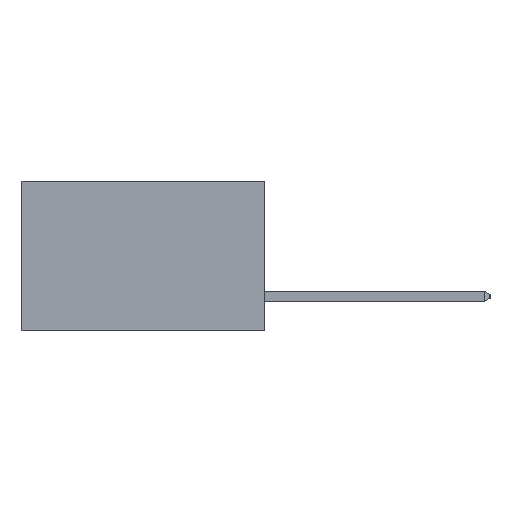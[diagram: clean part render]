
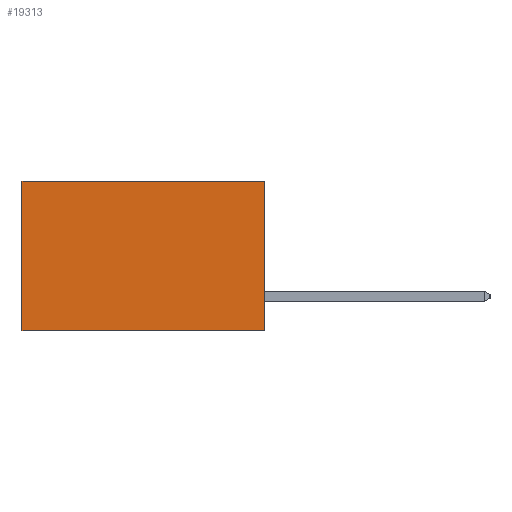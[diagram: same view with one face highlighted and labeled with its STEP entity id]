
A CAD part, left-side view. The second image highlights one B-rep face of the part: STEP entity #19313.
In plain terms, the highlighted planar face has unit normal (-1, 0, 0).
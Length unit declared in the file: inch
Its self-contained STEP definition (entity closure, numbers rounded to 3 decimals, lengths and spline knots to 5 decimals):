
#347 = ORIENTED_EDGE ( 'NONE', *, *, #15034, .F. ) ;
#660 = CARTESIAN_POINT ( 'NONE',  ( 0.2615, 0., -0.37 ) ) ;
#1065 = CARTESIAN_POINT ( 'NONE',  ( 0.2615, 0., -0.37 ) ) ;
#1078 = LINE ( 'NONE', #9106, #4583 ) ;
#1661 = EDGE_LOOP ( 'NONE', ( #18837, #2017, #347, #2575 ) ) ;
#2017 = ORIENTED_EDGE ( 'NONE', *, *, #21626, .F. ) ;
#2575 = ORIENTED_EDGE ( 'NONE', *, *, #17788, .T. ) ;
#3589 = VERTEX_POINT ( 'NONE', #18928 ) ;
#3694 = CARTESIAN_POINT ( 'NONE',  ( 0.2615, 0., 0. ) ) ;
#4120 = PLANE ( 'NONE',  #16615 ) ;
#4200 = DIRECTION ( 'NONE',  ( 1., 0., 0. ) ) ;
#4490 = CARTESIAN_POINT ( 'NONE',  ( 0.2615, 0., -0.37 ) ) ;
#4583 = VECTOR ( 'NONE', #10877, 39.37008 ) ;
#5473 = CARTESIAN_POINT ( 'NONE',  ( 0.2615, 0., 0. ) ) ;
#8933 = VECTOR ( 'NONE', #14797, 39.37008 ) ;
#9106 = CARTESIAN_POINT ( 'NONE',  ( 0.2615, 0., -0.37 ) ) ;
#9468 = LINE ( 'NONE', #4490, #8933 ) ;
#9940 = CARTESIAN_POINT ( 'NONE',  ( 0.2615, 0.6, 0. ) ) ;
#10675 = VECTOR ( 'NONE', #12567, 39.37008 ) ;
#10877 = DIRECTION ( 'NONE',  ( 0., 0., -1. ) ) ;
#12567 = DIRECTION ( 'NONE',  ( 0., 0., -1. ) ) ;
#13395 = VERTEX_POINT ( 'NONE', #3694 ) ;
#13861 = VERTEX_POINT ( 'NONE', #1065 ) ;
#14797 = DIRECTION ( 'NONE',  ( 0., 1., 0. ) ) ;
#15034 = EDGE_CURVE ( 'NONE', #13395, #13861, #1078, .T. ) ;
#15559 = LINE ( 'NONE', #5473, #19456 ) ;
#15735 = LINE ( 'NONE', #20854, #10675 ) ;
#16218 = DIRECTION ( 'NONE',  ( 0., 0., -1. ) ) ;
#16615 = AXIS2_PLACEMENT_3D ( 'NONE', #660, #4200, #16218 ) ;
#17788 = EDGE_CURVE ( 'NONE', #13395, #18881, #15559, .T. ) ;
#18837 = ORIENTED_EDGE ( 'NONE', *, *, #19802, .T. ) ;
#18881 = VERTEX_POINT ( 'NONE', #9940 ) ;
#18928 = CARTESIAN_POINT ( 'NONE',  ( 0.2615, 0.6, -0.37 ) ) ;
#19113 = DIRECTION ( 'NONE',  ( 0., 1., 0. ) ) ;
#19313 = ADVANCED_FACE ( 'NONE', ( #20130 ), #4120, .F. ) ;
#19456 = VECTOR ( 'NONE', #19113, 39.37008 ) ;
#19802 = EDGE_CURVE ( 'NONE', #18881, #3589, #15735, .T. ) ;
#20130 = FACE_OUTER_BOUND ( 'NONE', #1661, .T. ) ;
#20854 = CARTESIAN_POINT ( 'NONE',  ( 0.2615, 0.6, -0.37 ) ) ;
#21626 = EDGE_CURVE ( 'NONE', #13861, #3589, #9468, .T. ) ;
